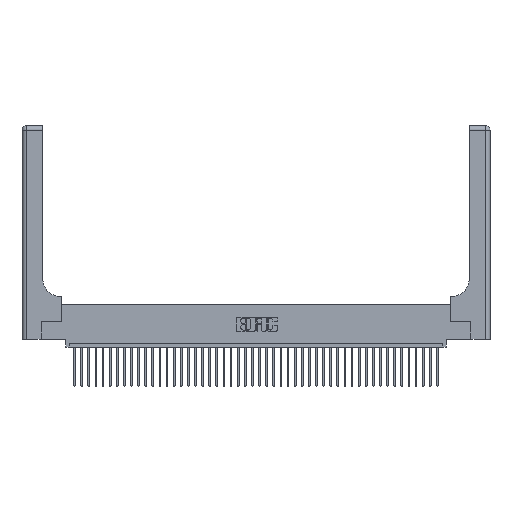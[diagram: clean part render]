
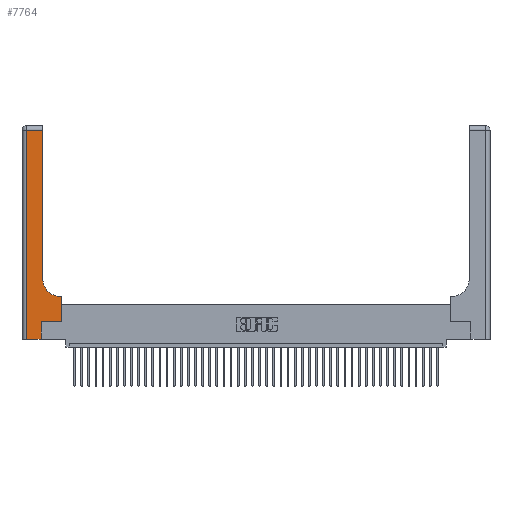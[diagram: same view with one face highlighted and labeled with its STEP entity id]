
A CAD part, top view. The second image highlights one B-rep face of the part: STEP entity #7764.
In plain terms, the highlighted planar face has unit normal (0, 0, 1).
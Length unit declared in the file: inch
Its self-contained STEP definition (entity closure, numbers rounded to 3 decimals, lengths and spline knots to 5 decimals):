
#1352 = LINE ( 'NONE', #28998, #35704 ) ;
#1829 = CARTESIAN_POINT ( 'NONE',  ( 0.06, 2.94, 0.37 ) ) ;
#2354 = DIRECTION ( 'NONE',  ( 0., 1., 0. ) ) ;
#2432 = LINE ( 'NONE', #35863, #34712 ) ;
#2437 = CARTESIAN_POINT ( 'NONE',  ( 0.269, 0., 0.37 ) ) ;
#3633 = ORIENTED_EDGE ( 'NONE', *, *, #10583, .T. ) ;
#4335 = DIRECTION ( 'NONE',  ( 0., -1., 0. ) ) ;
#5688 = CARTESIAN_POINT ( 'NONE',  ( 0.2915, 3., 0.37 ) ) ;
#5933 = EDGE_CURVE ( 'NONE', #9923, #39810, #32119, .T. ) ;
#7260 = VERTEX_POINT ( 'NONE', #36832 ) ;
#7510 = ORIENTED_EDGE ( 'NONE', *, *, #5933, .T. ) ;
#7715 = DIRECTION ( 'NONE',  ( 0., 0., -1. ) ) ;
#7764 = ADVANCED_FACE ( 'NONE', ( #31710 ), #22129, .F. ) ;
#8007 = VERTEX_POINT ( 'NONE', #16963 ) ;
#8493 = EDGE_CURVE ( 'NONE', #17212, #7260, #2432, .T. ) ;
#8659 = AXIS2_PLACEMENT_3D ( 'NONE', #25490, #28571, #11931 ) ;
#9321 = CARTESIAN_POINT ( 'NONE',  ( 0., 2.94, 0.37 ) ) ;
#9419 = CARTESIAN_POINT ( 'NONE',  ( 0.5585, 0.25, 0.37 ) ) ;
#9923 = VERTEX_POINT ( 'NONE', #35397 ) ;
#10583 = EDGE_CURVE ( 'NONE', #7260, #37658, #22050, .T. ) ;
#10625 = LINE ( 'NONE', #38807, #39263 ) ;
#11931 = DIRECTION ( 'NONE',  ( -1., 0., 0. ) ) ;
#12136 = VECTOR ( 'NONE', #12636, 39.37008 ) ;
#12392 = EDGE_CURVE ( 'NONE', #8007, #21020, #29752, .T. ) ;
#12636 = DIRECTION ( 'NONE',  ( 0., 1., 0. ) ) ;
#13032 = ORIENTED_EDGE ( 'NONE', *, *, #37429, .T. ) ;
#13349 = DIRECTION ( 'NONE',  ( 0., 1., 0. ) ) ;
#14112 = VECTOR ( 'NONE', #13349, 39.37008 ) ;
#15547 = DIRECTION ( 'NONE',  ( -1., 0., 0. ) ) ;
#16963 = CARTESIAN_POINT ( 'NONE',  ( 0.5585, 0.25, 0.37 ) ) ;
#17212 = VERTEX_POINT ( 'NONE', #20590 ) ;
#17600 = CARTESIAN_POINT ( 'NONE',  ( 0.5415, 0.85, 0.37 ) ) ;
#17843 = EDGE_CURVE ( 'NONE', #36990, #9923, #33761, .T. ) ;
#18853 = ORIENTED_EDGE ( 'NONE', *, *, #17843, .T. ) ;
#19497 = EDGE_CURVE ( 'NONE', #21020, #36990, #1352, .T. ) ;
#20523 = ORIENTED_EDGE ( 'NONE', *, *, #35888, .T. ) ;
#20590 = CARTESIAN_POINT ( 'NONE',  ( 0.06, 0., 0.37 ) ) ;
#21020 = VERTEX_POINT ( 'NONE', #40033 ) ;
#22050 = LINE ( 'NONE', #2437, #12136 ) ;
#22129 = PLANE ( 'NONE',  #8659 ) ;
#23389 = AXIS2_PLACEMENT_3D ( 'NONE', #17600, #7715, #41043 ) ;
#24050 = VECTOR ( 'NONE', #26097, 39.37008 ) ;
#24575 = CARTESIAN_POINT ( 'NONE',  ( 0.06, 3., 0.37 ) ) ;
#25490 = CARTESIAN_POINT ( 'NONE',  ( 0., 3., 0.37 ) ) ;
#26097 = DIRECTION ( 'NONE',  ( -1., 0., 0. ) ) ;
#28246 = ORIENTED_EDGE ( 'NONE', *, *, #19497, .T. ) ;
#28571 = DIRECTION ( 'NONE',  ( 0., 0., -1. ) ) ;
#28998 = CARTESIAN_POINT ( 'NONE',  ( 0.2915, 0.6, 0.37 ) ) ;
#29348 = VECTOR ( 'NONE', #4335, 39.37008 ) ;
#29752 = LINE ( 'NONE', #9419, #14112 ) ;
#30095 = EDGE_LOOP ( 'NONE', ( #7510, #37511, #13032, #42115, #3633, #20523, #40145, #28246, #18853 ) ) ;
#30577 = VECTOR ( 'NONE', #2354, 39.37008 ) ;
#31710 = FACE_OUTER_BOUND ( 'NONE', #30095, .T. ) ;
#32119 = LINE ( 'NONE', #5688, #30577 ) ;
#32274 = CARTESIAN_POINT ( 'NONE',  ( 0.269, 0.25, 0.37 ) ) ;
#33761 = CIRCLE ( 'NONE', #23389, 0.25 ) ;
#33868 = CARTESIAN_POINT ( 'NONE',  ( 0.2915, 2.94, 0.37 ) ) ;
#34409 = LINE ( 'NONE', #9321, #24050 ) ;
#34712 = VECTOR ( 'NONE', #38640, 39.37008 ) ;
#35397 = CARTESIAN_POINT ( 'NONE',  ( 0.2915, 0.85, 0.37 ) ) ;
#35531 = LINE ( 'NONE', #24575, #29348 ) ;
#35704 = VECTOR ( 'NONE', #15547, 39.37008 ) ;
#35863 = CARTESIAN_POINT ( 'NONE',  ( 0., 0., 0.37 ) ) ;
#35888 = EDGE_CURVE ( 'NONE', #37658, #8007, #10625, .T. ) ;
#36832 = CARTESIAN_POINT ( 'NONE',  ( 0.269, 0., 0.37 ) ) ;
#36990 = VERTEX_POINT ( 'NONE', #41901 ) ;
#37429 = EDGE_CURVE ( 'NONE', #37473, #17212, #35531, .T. ) ;
#37473 = VERTEX_POINT ( 'NONE', #1829 ) ;
#37511 = ORIENTED_EDGE ( 'NONE', *, *, #38251, .T. ) ;
#37658 = VERTEX_POINT ( 'NONE', #32274 ) ;
#38251 = EDGE_CURVE ( 'NONE', #39810, #37473, #34409, .T. ) ;
#38640 = DIRECTION ( 'NONE',  ( 1., 0., 0. ) ) ;
#38807 = CARTESIAN_POINT ( 'NONE',  ( 0.269, 0.25, 0.37 ) ) ;
#39263 = VECTOR ( 'NONE', #41747, 39.37008 ) ;
#39810 = VERTEX_POINT ( 'NONE', #33868 ) ;
#40033 = CARTESIAN_POINT ( 'NONE',  ( 0.5585, 0.6, 0.37 ) ) ;
#40145 = ORIENTED_EDGE ( 'NONE', *, *, #12392, .T. ) ;
#41043 = DIRECTION ( 'NONE',  ( 1., 0., 0. ) ) ;
#41747 = DIRECTION ( 'NONE',  ( 1., 0., 0. ) ) ;
#41901 = CARTESIAN_POINT ( 'NONE',  ( 0.5415, 0.6, 0.37 ) ) ;
#42115 = ORIENTED_EDGE ( 'NONE', *, *, #8493, .T. ) ;
